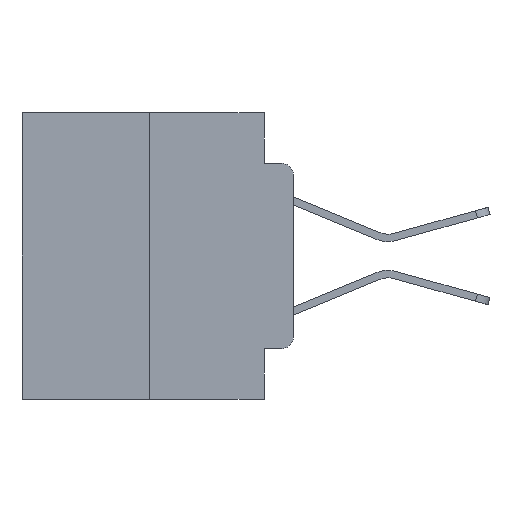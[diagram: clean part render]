
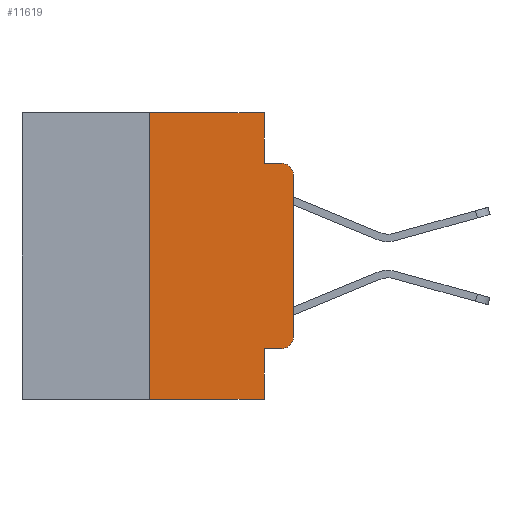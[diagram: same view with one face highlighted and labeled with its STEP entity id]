
A CAD part, left-side view. The second image highlights one B-rep face of the part: STEP entity #11619.
In plain terms, the highlighted planar face has unit normal (-1, 0, 0).
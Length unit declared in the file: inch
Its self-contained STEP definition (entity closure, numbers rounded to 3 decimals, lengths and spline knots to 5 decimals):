
#262 = LINE ( 'NONE', #23162, #14775 ) ;
#1480 = EDGE_CURVE ( 'NONE', #21726, #21271, #23431, .T. ) ;
#1524 = DIRECTION ( 'NONE',  ( -1., 0., 0. ) ) ;
#1535 = VERTEX_POINT ( 'NONE', #1643 ) ;
#1561 = CARTESIAN_POINT ( 'NONE',  ( 0., 0.051, -0.5 ) ) ;
#1643 = CARTESIAN_POINT ( 'NONE',  ( 0., 0., -0.3915 ) ) ;
#1788 = PLANE ( 'NONE',  #7644 ) ;
#1938 = LINE ( 'NONE', #25886, #4298 ) ;
#2309 = VECTOR ( 'NONE', #18001, 39.37008 ) ;
#2689 = VERTEX_POINT ( 'NONE', #2703 ) ;
#2703 = CARTESIAN_POINT ( 'NONE',  ( 0., 0., -0.1085 ) ) ;
#3246 = CARTESIAN_POINT ( 'NONE',  ( 0., 0.051, -0.4115 ) ) ;
#3766 = DIRECTION ( 'NONE',  ( 0., 0., -1. ) ) ;
#4053 = LINE ( 'NONE', #3246, #20903 ) ;
#4298 = VECTOR ( 'NONE', #8298, 39.37008 ) ;
#4472 = VERTEX_POINT ( 'NONE', #15398 ) ;
#4856 = VERTEX_POINT ( 'NONE', #27717 ) ;
#5418 = DIRECTION ( 'NONE',  ( 0., -1., 0. ) ) ;
#5694 = DIRECTION ( 'NONE',  ( -1., 0., 0. ) ) ;
#5949 = DIRECTION ( 'NONE',  ( 1., 0., 0. ) ) ;
#6515 = EDGE_CURVE ( 'NONE', #27440, #6646, #25303, .T. ) ;
#6646 = VERTEX_POINT ( 'NONE', #24758 ) ;
#7347 = EDGE_CURVE ( 'NONE', #21726, #27440, #26243, .T. ) ;
#7644 = AXIS2_PLACEMENT_3D ( 'NONE', #14815, #5949, #3766 ) ;
#7771 = ORIENTED_EDGE ( 'NONE', *, *, #1480, .T. ) ;
#7809 = VECTOR ( 'NONE', #11292, 39.37008 ) ;
#8034 = EDGE_CURVE ( 'NONE', #22024, #4472, #262, .T. ) ;
#8137 = EDGE_CURVE ( 'NONE', #6646, #22024, #1938, .T. ) ;
#8298 = DIRECTION ( 'NONE',  ( 0., 0., -1. ) ) ;
#8364 = EDGE_CURVE ( 'NONE', #1535, #2689, #24543, .T. ) ;
#8886 = ORIENTED_EDGE ( 'NONE', *, *, #24463, .T. ) ;
#8984 = VERTEX_POINT ( 'NONE', #14208 ) ;
#10533 = CIRCLE ( 'NONE', #20074, 0.02 ) ;
#10674 = ORIENTED_EDGE ( 'NONE', *, *, #6515, .F. ) ;
#11242 = ORIENTED_EDGE ( 'NONE', *, *, #8137, .F. ) ;
#11292 = DIRECTION ( 'NONE',  ( 0., -1., 0. ) ) ;
#11601 = ORIENTED_EDGE ( 'NONE', *, *, #7347, .F. ) ;
#11619 = ADVANCED_FACE ( 'NONE', ( #18302 ), #1788, .F. ) ;
#12400 = EDGE_CURVE ( 'NONE', #4856, #1535, #10533, .T. ) ;
#12523 = CARTESIAN_POINT ( 'NONE',  ( 0., 0.473, -0.5 ) ) ;
#13165 = CARTESIAN_POINT ( 'NONE',  ( 0., 0.051, 0. ) ) ;
#13187 = VECTOR ( 'NONE', #19825, 39.37008 ) ;
#13554 = ORIENTED_EDGE ( 'NONE', *, *, #8364, .T. ) ;
#13824 = EDGE_LOOP ( 'NONE', ( #13554, #15660, #14861, #11242, #10674, #11601, #7771, #21916, #8886, #21803 ) ) ;
#14208 = CARTESIAN_POINT ( 'NONE',  ( 0., 0.051, -0.4115 ) ) ;
#14775 = VECTOR ( 'NONE', #20787, 39.37008 ) ;
#14815 = CARTESIAN_POINT ( 'NONE',  ( 0., 0.473, 0. ) ) ;
#14861 = ORIENTED_EDGE ( 'NONE', *, *, #8034, .F. ) ;
#15311 = CARTESIAN_POINT ( 'NONE',  ( 0., 0.473, 0. ) ) ;
#15398 = CARTESIAN_POINT ( 'NONE',  ( 0., 0.02, -0.0885 ) ) ;
#15630 = CARTESIAN_POINT ( 'NONE',  ( 0., 0., 0. ) ) ;
#15660 = ORIENTED_EDGE ( 'NONE', *, *, #19553, .T. ) ;
#15869 = CARTESIAN_POINT ( 'NONE',  ( 0., 0.25, 0. ) ) ;
#16342 = DIRECTION ( 'NONE',  ( 0., 0., -1. ) ) ;
#16520 = LINE ( 'NONE', #13165, #13187 ) ;
#16717 = AXIS2_PLACEMENT_3D ( 'NONE', #17067, #1524, #25736 ) ;
#17067 = CARTESIAN_POINT ( 'NONE',  ( 0., 0.02, -0.1085 ) ) ;
#17579 = DIRECTION ( 'NONE',  ( 0., 0., 1. ) ) ;
#17752 = VECTOR ( 'NONE', #17579, 39.37008 ) ;
#18001 = DIRECTION ( 'NONE',  ( 0., 0., 1. ) ) ;
#18302 = FACE_OUTER_BOUND ( 'NONE', #13824, .T. ) ;
#18404 = CARTESIAN_POINT ( 'NONE',  ( 0., 0.02, -0.3915 ) ) ;
#19553 = EDGE_CURVE ( 'NONE', #2689, #4472, #23188, .T. ) ;
#19825 = DIRECTION ( 'NONE',  ( 0., 0., -1. ) ) ;
#20074 = AXIS2_PLACEMENT_3D ( 'NONE', #18404, #5694, #16342 ) ;
#20787 = DIRECTION ( 'NONE',  ( 0., -1., 0. ) ) ;
#20903 = VECTOR ( 'NONE', #5418, 39.37008 ) ;
#21141 = DIRECTION ( 'NONE',  ( 0., -1., 0. ) ) ;
#21271 = VERTEX_POINT ( 'NONE', #1561 ) ;
#21726 = VERTEX_POINT ( 'NONE', #24469 ) ;
#21803 = ORIENTED_EDGE ( 'NONE', *, *, #12400, .T. ) ;
#21916 = ORIENTED_EDGE ( 'NONE', *, *, #24803, .F. ) ;
#22024 = VERTEX_POINT ( 'NONE', #27260 ) ;
#23100 = VECTOR ( 'NONE', #21141, 39.37008 ) ;
#23162 = CARTESIAN_POINT ( 'NONE',  ( 0., 0.051, -0.0885 ) ) ;
#23188 = CIRCLE ( 'NONE', #16717, 0.02 ) ;
#23431 = LINE ( 'NONE', #12523, #23100 ) ;
#24463 = EDGE_CURVE ( 'NONE', #8984, #4856, #4053, .T. ) ;
#24469 = CARTESIAN_POINT ( 'NONE',  ( 0., 0.25, -0.5 ) ) ;
#24543 = LINE ( 'NONE', #15630, #17752 ) ;
#24758 = CARTESIAN_POINT ( 'NONE',  ( 0., 0.051, 0. ) ) ;
#24803 = EDGE_CURVE ( 'NONE', #8984, #21271, #16520, .T. ) ;
#25303 = LINE ( 'NONE', #15311, #7809 ) ;
#25419 = CARTESIAN_POINT ( 'NONE',  ( 0., 0.25, 0. ) ) ;
#25736 = DIRECTION ( 'NONE',  ( 0., 0., -1. ) ) ;
#25886 = CARTESIAN_POINT ( 'NONE',  ( 0., 0.051, 0. ) ) ;
#26243 = LINE ( 'NONE', #15869, #2309 ) ;
#27260 = CARTESIAN_POINT ( 'NONE',  ( 0., 0.051, -0.0885 ) ) ;
#27440 = VERTEX_POINT ( 'NONE', #25419 ) ;
#27717 = CARTESIAN_POINT ( 'NONE',  ( 0., 0.02, -0.4115 ) ) ;
